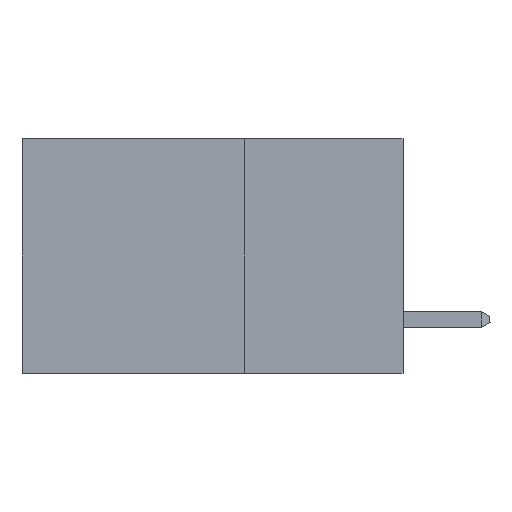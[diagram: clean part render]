
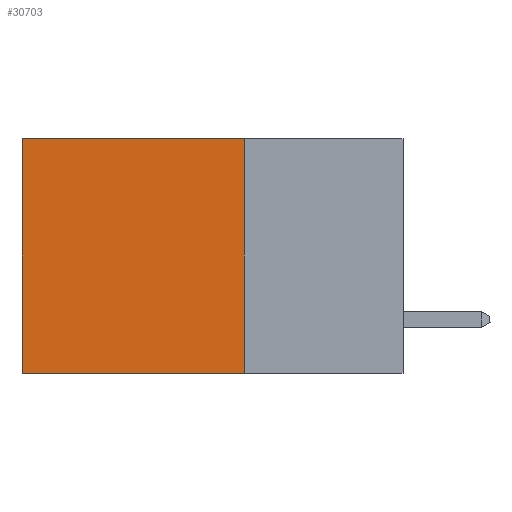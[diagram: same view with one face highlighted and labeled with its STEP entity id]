
A CAD part, left-side view. The second image highlights one B-rep face of the part: STEP entity #30703.
In plain terms, the highlighted planar face has unit normal (-1, 0, 0).
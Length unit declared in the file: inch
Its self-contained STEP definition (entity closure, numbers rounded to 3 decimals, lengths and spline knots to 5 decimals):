
#123 = EDGE_CURVE ( 'NONE', #6681, #1069, #28833, .T. ) ;
#1069 = VERTEX_POINT ( 'NONE', #21760 ) ;
#3336 = PLANE ( 'NONE',  #40517 ) ;
#4021 = VECTOR ( 'NONE', #31278, 39.37008 ) ;
#4674 = EDGE_CURVE ( 'NONE', #16045, #6681, #23660, .T. ) ;
#5632 = CARTESIAN_POINT ( 'NONE',  ( 0.2875, 0.25, -0.37 ) ) ;
#5738 = VECTOR ( 'NONE', #27534, 39.37008 ) ;
#6544 = CARTESIAN_POINT ( 'NONE',  ( 0.2875, 0.6, 0. ) ) ;
#6681 = VERTEX_POINT ( 'NONE', #21022 ) ;
#6855 = LINE ( 'NONE', #36823, #5738 ) ;
#7492 = EDGE_LOOP ( 'NONE', ( #31311, #11645, #26284, #7637 ) ) ;
#7637 = ORIENTED_EDGE ( 'NONE', *, *, #4674, .T. ) ;
#11645 = ORIENTED_EDGE ( 'NONE', *, *, #28761, .F. ) ;
#11730 = VERTEX_POINT ( 'NONE', #38120 ) ;
#16045 = VERTEX_POINT ( 'NONE', #42680 ) ;
#16931 = VECTOR ( 'NONE', #21064, 39.37008 ) ;
#17813 = CARTESIAN_POINT ( 'NONE',  ( 0.2875, 0.25, 0. ) ) ;
#18709 = EDGE_CURVE ( 'NONE', #16045, #11730, #6855, .T. ) ;
#20501 = DIRECTION ( 'NONE',  ( 1., 0., 0. ) ) ;
#21022 = CARTESIAN_POINT ( 'NONE',  ( 0.2875, 0.6, 0. ) ) ;
#21064 = DIRECTION ( 'NONE',  ( 0., 0., -1. ) ) ;
#21760 = CARTESIAN_POINT ( 'NONE',  ( 0.2875, 0.6, -0.37 ) ) ;
#22892 = FACE_OUTER_BOUND ( 'NONE', #7492, .T. ) ;
#23660 = LINE ( 'NONE', #17813, #4021 ) ;
#26284 = ORIENTED_EDGE ( 'NONE', *, *, #18709, .F. ) ;
#27534 = DIRECTION ( 'NONE',  ( 0., 0., -1. ) ) ;
#27963 = LINE ( 'NONE', #5632, #36697 ) ;
#28761 = EDGE_CURVE ( 'NONE', #11730, #1069, #27963, .T. ) ;
#28833 = LINE ( 'NONE', #6544, #16931 ) ;
#29639 = DIRECTION ( 'NONE',  ( 0., 1., 0. ) ) ;
#30703 = ADVANCED_FACE ( 'NONE', ( #22892 ), #3336, .F. ) ;
#31008 = DIRECTION ( 'NONE',  ( 0., 0., -1. ) ) ;
#31190 = CARTESIAN_POINT ( 'NONE',  ( 0.2875, 0.25, 0. ) ) ;
#31278 = DIRECTION ( 'NONE',  ( 0., 1., 0. ) ) ;
#31311 = ORIENTED_EDGE ( 'NONE', *, *, #123, .T. ) ;
#36697 = VECTOR ( 'NONE', #29639, 39.37008 ) ;
#36823 = CARTESIAN_POINT ( 'NONE',  ( 0.2875, 0.25, 0. ) ) ;
#38120 = CARTESIAN_POINT ( 'NONE',  ( 0.2875, 0.25, -0.37 ) ) ;
#40517 = AXIS2_PLACEMENT_3D ( 'NONE', #31190, #20501, #31008 ) ;
#42680 = CARTESIAN_POINT ( 'NONE',  ( 0.2875, 0.25, 0. ) ) ;
